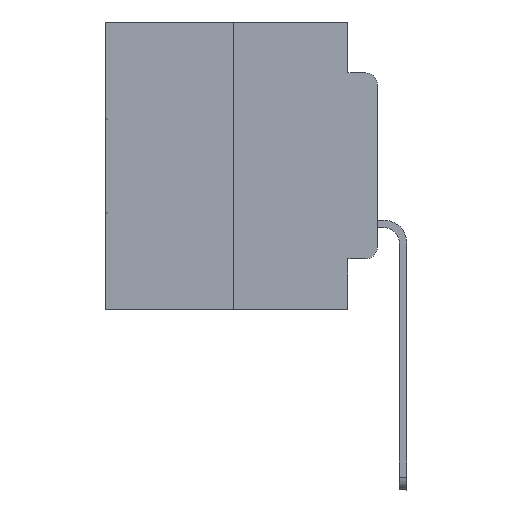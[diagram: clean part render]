
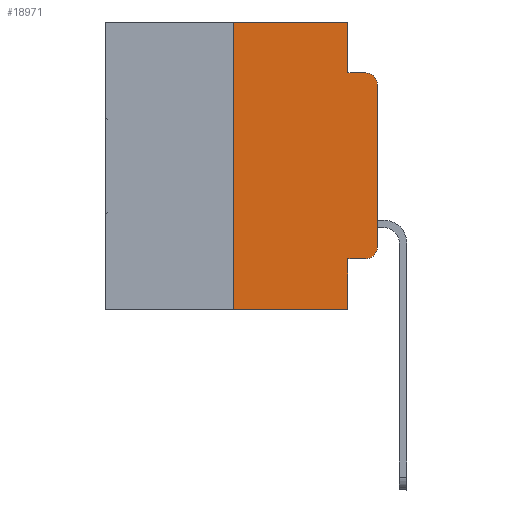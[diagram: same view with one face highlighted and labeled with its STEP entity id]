
A CAD part, left-side view. The second image highlights one B-rep face of the part: STEP entity #18971.
In plain terms, the highlighted planar face has unit normal (-1, 0, 0).
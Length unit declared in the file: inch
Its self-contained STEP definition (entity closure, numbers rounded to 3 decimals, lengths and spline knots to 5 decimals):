
#62 = DIRECTION ( 'NONE',  ( 0., -1., 0. ) ) ;
#67 = FACE_OUTER_BOUND ( 'NONE', #21989, .T. ) ;
#75 = CARTESIAN_POINT ( 'NONE',  ( 0., 0.051, 0. ) ) ;
#197 = LINE ( 'NONE', #9874, #15114 ) ;
#678 = AXIS2_PLACEMENT_3D ( 'NONE', #4990, #7512, #22114 ) ;
#1144 = VECTOR ( 'NONE', #28649, 39.37008 ) ;
#1148 = DIRECTION ( 'NONE',  ( -1., 0., 0. ) ) ;
#1292 = CARTESIAN_POINT ( 'NONE',  ( 0., 0.02, -0.3915 ) ) ;
#1387 = AXIS2_PLACEMENT_3D ( 'NONE', #1292, #1148, #30211 ) ;
#1878 = CARTESIAN_POINT ( 'NONE',  ( 0., 0.473, 0. ) ) ;
#2494 = EDGE_CURVE ( 'NONE', #18821, #10606, #11177, .T. ) ;
#2536 = EDGE_CURVE ( 'NONE', #22751, #8718, #14176, .T. ) ;
#2619 = DIRECTION ( 'NONE',  ( -1., 0., 0. ) ) ;
#2632 = ORIENTED_EDGE ( 'NONE', *, *, #5855, .F. ) ;
#2806 = DIRECTION ( 'NONE',  ( 0., 0., 1. ) ) ;
#3422 = VERTEX_POINT ( 'NONE', #29006 ) ;
#3819 = CARTESIAN_POINT ( 'NONE',  ( 0., 0.051, -0.0885 ) ) ;
#4092 = ORIENTED_EDGE ( 'NONE', *, *, #24855, .F. ) ;
#4352 = CARTESIAN_POINT ( 'NONE',  ( 0., 0.473, -0.5 ) ) ;
#4406 = CIRCLE ( 'NONE', #1387, 0.02 ) ;
#4920 = CARTESIAN_POINT ( 'NONE',  ( 0., 0.02, -0.4115 ) ) ;
#4936 = CARTESIAN_POINT ( 'NONE',  ( 0., 0., -0.3915 ) ) ;
#4990 = CARTESIAN_POINT ( 'NONE',  ( 0., 0.473, 0. ) ) ;
#5221 = CARTESIAN_POINT ( 'NONE',  ( 0., 0.25, -0.5 ) ) ;
#5855 = EDGE_CURVE ( 'NONE', #10606, #20857, #16178, .T. ) ;
#7220 = VERTEX_POINT ( 'NONE', #4936 ) ;
#7512 = DIRECTION ( 'NONE',  ( 1., 0., 0. ) ) ;
#7926 = EDGE_CURVE ( 'NONE', #27232, #18362, #12784, .T. ) ;
#8627 = ORIENTED_EDGE ( 'NONE', *, *, #18898, .T. ) ;
#8718 = VERTEX_POINT ( 'NONE', #4920 ) ;
#8992 = LINE ( 'NONE', #23113, #12530 ) ;
#9303 = DIRECTION ( 'NONE',  ( 0., -1., 0. ) ) ;
#9757 = CARTESIAN_POINT ( 'NONE',  ( 0., 0.02, -0.1085 ) ) ;
#9874 = CARTESIAN_POINT ( 'NONE',  ( 0., 0.051, 0. ) ) ;
#10282 = CARTESIAN_POINT ( 'NONE',  ( 0., 0.25, 0. ) ) ;
#10606 = VERTEX_POINT ( 'NONE', #10282 ) ;
#10633 = CARTESIAN_POINT ( 'NONE',  ( 0., 0.02, -0.0885 ) ) ;
#11177 = LINE ( 'NONE', #20859, #28786 ) ;
#11491 = LINE ( 'NONE', #4352, #1144 ) ;
#11827 = EDGE_CURVE ( 'NONE', #8718, #7220, #4406, .T. ) ;
#12304 = DIRECTION ( 'NONE',  ( 0., 0., -1. ) ) ;
#12530 = VECTOR ( 'NONE', #9303, 39.37008 ) ;
#12784 = CIRCLE ( 'NONE', #23413, 0.02 ) ;
#13107 = VECTOR ( 'NONE', #16482, 39.37008 ) ;
#14076 = LINE ( 'NONE', #21529, #27433 ) ;
#14176 = LINE ( 'NONE', #26413, #21150 ) ;
#14224 = CARTESIAN_POINT ( 'NONE',  ( 0., 0.051, 0. ) ) ;
#15114 = VECTOR ( 'NONE', #21453, 39.37008 ) ;
#15132 = VECTOR ( 'NONE', #31403, 39.37008 ) ;
#15151 = ORIENTED_EDGE ( 'NONE', *, *, #2494, .F. ) ;
#15406 = EDGE_CURVE ( 'NONE', #7220, #27232, #14076, .T. ) ;
#16178 = LINE ( 'NONE', #1878, #13107 ) ;
#16482 = DIRECTION ( 'NONE',  ( 0., -1., 0. ) ) ;
#16897 = ORIENTED_EDGE ( 'NONE', *, *, #25900, .F. ) ;
#17631 = CARTESIAN_POINT ( 'NONE',  ( 0., 0., -0.1085 ) ) ;
#18362 = VERTEX_POINT ( 'NONE', #10633 ) ;
#18478 = DIRECTION ( 'NONE',  ( 0., 0., 1. ) ) ;
#18821 = VERTEX_POINT ( 'NONE', #5221 ) ;
#18898 = EDGE_CURVE ( 'NONE', #18821, #3422, #11491, .T. ) ;
#18971 = ADVANCED_FACE ( 'NONE', ( #67 ), #29286, .F. ) ;
#18972 = ORIENTED_EDGE ( 'NONE', *, *, #29504, .F. ) ;
#19314 = LINE ( 'NONE', #14224, #15132 ) ;
#20857 = VERTEX_POINT ( 'NONE', #75 ) ;
#20859 = CARTESIAN_POINT ( 'NONE',  ( 0., 0.25, 0. ) ) ;
#21001 = ORIENTED_EDGE ( 'NONE', *, *, #7926, .T. ) ;
#21150 = VECTOR ( 'NONE', #62, 39.37008 ) ;
#21453 = DIRECTION ( 'NONE',  ( 0., 0., -1. ) ) ;
#21529 = CARTESIAN_POINT ( 'NONE',  ( 0., 0., 0. ) ) ;
#21989 = EDGE_LOOP ( 'NONE', ( #22662, #21001, #4092, #16897, #2632, #15151, #8627, #18972, #25122, #28551 ) ) ;
#22114 = DIRECTION ( 'NONE',  ( 0., 0., -1. ) ) ;
#22662 = ORIENTED_EDGE ( 'NONE', *, *, #15406, .T. ) ;
#22751 = VERTEX_POINT ( 'NONE', #27509 ) ;
#23113 = CARTESIAN_POINT ( 'NONE',  ( 0., 0.051, -0.0885 ) ) ;
#23413 = AXIS2_PLACEMENT_3D ( 'NONE', #9757, #2619, #12304 ) ;
#24855 = EDGE_CURVE ( 'NONE', #27340, #18362, #8992, .T. ) ;
#25122 = ORIENTED_EDGE ( 'NONE', *, *, #2536, .T. ) ;
#25900 = EDGE_CURVE ( 'NONE', #20857, #27340, #197, .T. ) ;
#26413 = CARTESIAN_POINT ( 'NONE',  ( 0., 0.051, -0.4115 ) ) ;
#27232 = VERTEX_POINT ( 'NONE', #17631 ) ;
#27340 = VERTEX_POINT ( 'NONE', #3819 ) ;
#27433 = VECTOR ( 'NONE', #2806, 39.37008 ) ;
#27509 = CARTESIAN_POINT ( 'NONE',  ( 0., 0.051, -0.4115 ) ) ;
#28551 = ORIENTED_EDGE ( 'NONE', *, *, #11827, .T. ) ;
#28649 = DIRECTION ( 'NONE',  ( 0., -1., 0. ) ) ;
#28786 = VECTOR ( 'NONE', #18478, 39.37008 ) ;
#29006 = CARTESIAN_POINT ( 'NONE',  ( 0., 0.051, -0.5 ) ) ;
#29286 = PLANE ( 'NONE',  #678 ) ;
#29504 = EDGE_CURVE ( 'NONE', #22751, #3422, #19314, .T. ) ;
#30211 = DIRECTION ( 'NONE',  ( 0., 0., -1. ) ) ;
#31403 = DIRECTION ( 'NONE',  ( 0., 0., -1. ) ) ;
